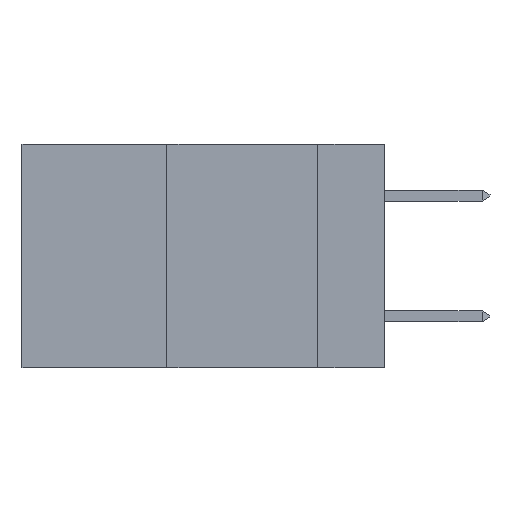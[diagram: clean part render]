
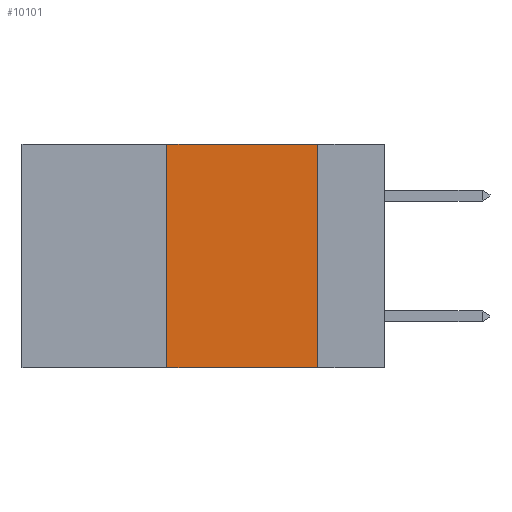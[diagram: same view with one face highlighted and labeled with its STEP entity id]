
A CAD part, left-side view. The second image highlights one B-rep face of the part: STEP entity #10101.
In plain terms, the highlighted planar face has unit normal (-1, 0, 0).
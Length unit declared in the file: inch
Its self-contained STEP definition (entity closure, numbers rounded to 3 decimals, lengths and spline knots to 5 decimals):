
#300 = CARTESIAN_POINT ( 'NONE',  ( 0., 0.36, -0.37 ) ) ;
#544 = CARTESIAN_POINT ( 'NONE',  ( 0., 0.11, -0.37 ) ) ;
#2075 = LINE ( 'NONE', #5914, #12866 ) ;
#2224 = EDGE_CURVE ( 'NONE', #3266, #6311, #6658, .T. ) ;
#2225 = DIRECTION ( 'NONE',  ( 0., -1., 0. ) ) ;
#2638 = FACE_OUTER_BOUND ( 'NONE', #3928, .T. ) ;
#2688 = ORIENTED_EDGE ( 'NONE', *, *, #12660, .F. ) ;
#2916 = CARTESIAN_POINT ( 'NONE',  ( 0., 0.6, -0.37 ) ) ;
#3038 = LINE ( 'NONE', #4682, #12475 ) ;
#3235 = ORIENTED_EDGE ( 'NONE', *, *, #2224, .T. ) ;
#3266 = VERTEX_POINT ( 'NONE', #300 ) ;
#3541 = DIRECTION ( 'NONE',  ( 1., 0., 0. ) ) ;
#3928 = EDGE_LOOP ( 'NONE', ( #2688, #7414, #12059, #3235 ) ) ;
#4017 = DIRECTION ( 'NONE',  ( 0., -1., 0. ) ) ;
#4682 = CARTESIAN_POINT ( 'NONE',  ( 0., 0.11, 0. ) ) ;
#5055 = VERTEX_POINT ( 'NONE', #5235 ) ;
#5228 = EDGE_CURVE ( 'NONE', #9153, #5055, #11381, .T. ) ;
#5235 = CARTESIAN_POINT ( 'NONE',  ( 0., 0.11, 0. ) ) ;
#5914 = CARTESIAN_POINT ( 'NONE',  ( 0., 0.36, 0. ) ) ;
#6311 = VERTEX_POINT ( 'NONE', #544 ) ;
#6430 = VECTOR ( 'NONE', #2225, 39.37008 ) ;
#6602 = EDGE_CURVE ( 'NONE', #3266, #9153, #2075, .T. ) ;
#6658 = LINE ( 'NONE', #2916, #8148 ) ;
#7414 = ORIENTED_EDGE ( 'NONE', *, *, #5228, .F. ) ;
#8148 = VECTOR ( 'NONE', #4017, 39.37008 ) ;
#8290 = CARTESIAN_POINT ( 'NONE',  ( 0., 0.6, 0. ) ) ;
#9153 = VERTEX_POINT ( 'NONE', #13040 ) ;
#9832 = PLANE ( 'NONE',  #13402 ) ;
#9917 = DIRECTION ( 'NONE',  ( 0., 0., -1. ) ) ;
#10101 = ADVANCED_FACE ( 'NONE', ( #2638 ), #9832, .F. ) ;
#11381 = LINE ( 'NONE', #8290, #6430 ) ;
#11877 = DIRECTION ( 'NONE',  ( 0., 0., -1. ) ) ;
#12059 = ORIENTED_EDGE ( 'NONE', *, *, #6602, .F. ) ;
#12252 = DIRECTION ( 'NONE',  ( 0., 0., 1. ) ) ;
#12475 = VECTOR ( 'NONE', #11877, 39.37008 ) ;
#12660 = EDGE_CURVE ( 'NONE', #5055, #6311, #3038, .T. ) ;
#12866 = VECTOR ( 'NONE', #12252, 39.37008 ) ;
#12938 = CARTESIAN_POINT ( 'NONE',  ( 0., 0.6, 0. ) ) ;
#13040 = CARTESIAN_POINT ( 'NONE',  ( 0., 0.36, 0. ) ) ;
#13402 = AXIS2_PLACEMENT_3D ( 'NONE', #12938, #3541, #9917 ) ;
